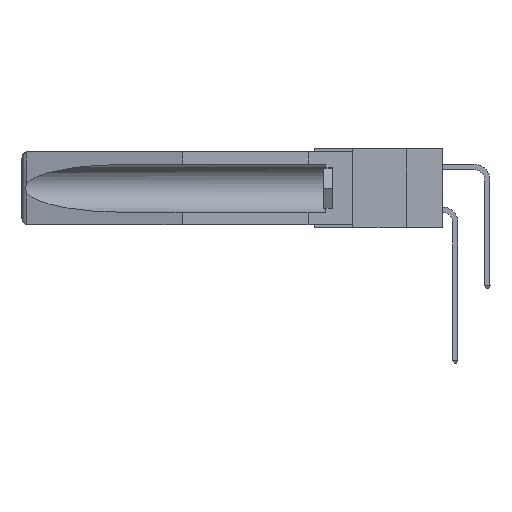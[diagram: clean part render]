
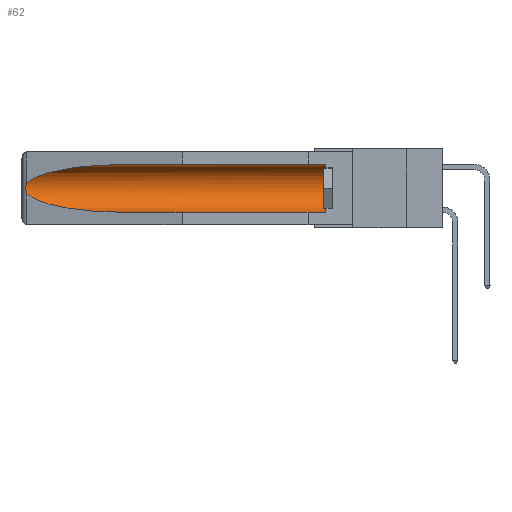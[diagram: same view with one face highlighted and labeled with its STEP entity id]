
A CAD part, left-side view. The second image highlights one B-rep face of the part: STEP entity #62.
In plain terms, the highlighted cylindrical face has radius 2.857 mm (diameter 5.715 mm), a partial arc.
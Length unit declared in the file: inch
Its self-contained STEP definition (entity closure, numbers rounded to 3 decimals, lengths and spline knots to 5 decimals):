
#62 = ADVANCED_FACE ( 'NONE', ( #3431 ), #166, .F. ) ;
#166 = CYLINDRICAL_SURFACE ( 'NONE', #1702, 0.1125 ) ;
#498 = CARTESIAN_POINT ( 'NONE',  ( 0.155, 1.07973, -0.059 ) ) ;
#568 = CARTESIAN_POINT ( 'NONE',  ( 0.25451, 1.48313, -0.09465 ) ) ;
#830 = ORIENTED_EDGE ( 'NONE', *, *, #23297, .T. ) ;
#1090 = ORIENTED_EDGE ( 'NONE', *, *, #8979, .F. ) ;
#1702 = AXIS2_PLACEMENT_3D ( 'NONE', #5433, #23674, #26337 ) ;
#2218 = CIRCLE ( 'NONE', #22630, 0.1125 ) ;
#3092 = VECTOR ( 'NONE', #3189, 39.37008 ) ;
#3189 = DIRECTION ( 'NONE',  ( 0., 1., 0. ) ) ;
#3304 = CARTESIAN_POINT ( 'NONE',  ( 0.26654, 1.53092, -0.15636 ) ) ;
#3431 = FACE_OUTER_BOUND ( 'NONE', #16667, .T. ) ;
#3472 = ORIENTED_EDGE ( 'NONE', *, *, #8042, .T. ) ;
#3806 = CARTESIAN_POINT ( 'NONE',  ( 0.155, 0.126, -0.284 ) ) ;
#5011 = ORIENTED_EDGE ( 'NONE', *, *, #14254, .T. ) ;
#5397 = DIRECTION ( 'NONE',  ( 0., -1., 0. ) ) ;
#5424 = VERTEX_POINT ( 'NONE', #498 ) ;
#5433 = CARTESIAN_POINT ( 'NONE',  ( 0.155, -0.30754, -0.1715 ) ) ;
#6238 = VERTEX_POINT ( 'NONE', #3806 ) ;
#7282 = EDGE_CURVE ( 'NONE', #6238, #15183, #2218, .T. ) ;
#7394 = CARTESIAN_POINT ( 'NONE',  ( 0.2675, 1.53308, -0.17534 ) ) ;
#7435 = CARTESIAN_POINT ( 'NONE',  ( 0.155, 0.126, -0.059 ) ) ;
#7618 = DIRECTION ( 'NONE',  ( 0., 0., 1. ) ) ;
#7759 = CARTESIAN_POINT ( 'NONE',  ( 0.26655, 1.53094, -0.18657 ) ) ;
#8042 = EDGE_CURVE ( 'NONE', #5424, #17426, #20047, .T. ) ;
#8227 = CARTESIAN_POINT ( 'NONE',  ( 0.26537, 1.52718, -0.14972 ) ) ;
#8979 = EDGE_CURVE ( 'NONE', #6238, #10886, #10139, .T. ) ;
#9926 = CARTESIAN_POINT ( 'NONE',  ( 0.26537, 1.52718, -0.19328 ) ) ;
#10139 = LINE ( 'NONE', #11407, #3092 ) ;
#10175 = CARTESIAN_POINT ( 'NONE',  ( 0.155, 1.07973, -0.284 ) ) ;
#10333 = CARTESIAN_POINT ( 'NONE',  ( 0.21114, 1.30732, -0.284 ) ) ;
#10658 = ORIENTED_EDGE ( 'NONE', *, *, #7282, .T. ) ;
#10886 = VERTEX_POINT ( 'NONE', #13370 ) ;
#11407 = CARTESIAN_POINT ( 'NONE',  ( 0.155, -0.30754, -0.284 ) ) ;
#11933 =( BOUNDED_CURVE ( )  B_SPLINE_CURVE ( 3, ( #24404, #22502, #10333, #10175 ),
 .UNSPECIFIED., .F., .F. ) 
 B_SPLINE_CURVE_WITH_KNOTS ( ( 4, 4 ),
 ( 0.1948, 1.5708 ),
 .UNSPECIFIED. ) 
 CURVE ( )  GEOMETRIC_REPRESENTATION_ITEM ( )  RATIONAL_B_SPLINE_CURVE ( ( 1., 0.848, 0.848, 1. ) ) 
 REPRESENTATION_ITEM ( '' )  );
#12112 = VERTEX_POINT ( 'NONE', #9926 ) ;
#12796 = ORIENTED_EDGE ( 'NONE', *, *, #21120, .T. ) ;
#13083 = B_SPLINE_CURVE_WITH_KNOTS ( 'NONE', 3,
 ( #24043, #19747, #3304, #17957, #21881, #7394, #21969, #7759, #25896, #23866 ),
 .UNSPECIFIED., .F., .F.,
 ( 4, 2, 2, 2, 4 ),
 ( 0., 0.00029, 0.00058, 0.00087, 0.00117 ),
 .UNSPECIFIED. ) ;
#13370 = CARTESIAN_POINT ( 'NONE',  ( 0.155, 1.07973, -0.284 ) ) ;
#14254 = EDGE_CURVE ( 'NONE', #12112, #10886, #11933, .T. ) ;
#14937 = CARTESIAN_POINT ( 'NONE',  ( 0.26537, 1.52718, -0.14972 ) ) ;
#15183 = VERTEX_POINT ( 'NONE', #7435 ) ;
#16667 = EDGE_LOOP ( 'NONE', ( #3472, #830, #5011, #1090, #10658, #12796 ) ) ;
#16756 = CARTESIAN_POINT ( 'NONE',  ( 0.155, 1.07973, -0.059 ) ) ;
#16911 = VECTOR ( 'NONE', #26166, 39.37008 ) ;
#17426 = VERTEX_POINT ( 'NONE', #8227 ) ;
#17957 = CARTESIAN_POINT ( 'NONE',  ( 0.2673, 1.5327, -0.16383 ) ) ;
#19747 = CARTESIAN_POINT ( 'NONE',  ( 0.26597, 1.52961, -0.15275 ) ) ;
#20047 =( BOUNDED_CURVE ( )  B_SPLINE_CURVE ( 3, ( #16756, #25010, #568, #14937 ),
 .UNSPECIFIED., .F., .F. ) 
 B_SPLINE_CURVE_WITH_KNOTS ( ( 4, 4 ),
 ( 4.71239, 6.08839 ),
 .UNSPECIFIED. ) 
 CURVE ( )  GEOMETRIC_REPRESENTATION_ITEM ( )  RATIONAL_B_SPLINE_CURVE ( ( 1., 0.848, 0.848, 1. ) ) 
 REPRESENTATION_ITEM ( '' )  );
#21120 = EDGE_CURVE ( 'NONE', #15183, #5424, #23973, .T. ) ;
#21881 = CARTESIAN_POINT ( 'NONE',  ( 0.2675, 1.53308, -0.16763 ) ) ;
#21915 = CARTESIAN_POINT ( 'NONE',  ( 0.155, 0.126, -0.1715 ) ) ;
#21969 = CARTESIAN_POINT ( 'NONE',  ( 0.2673, 1.53269, -0.17917 ) ) ;
#22322 = CARTESIAN_POINT ( 'NONE',  ( 0.155, -0.30754, -0.059 ) ) ;
#22502 = CARTESIAN_POINT ( 'NONE',  ( 0.25451, 1.48313, -0.24835 ) ) ;
#22630 = AXIS2_PLACEMENT_3D ( 'NONE', #21915, #5397, #7618 ) ;
#23297 = EDGE_CURVE ( 'NONE', #17426, #12112, #13083, .T. ) ;
#23674 = DIRECTION ( 'NONE',  ( 0., 1., 0. ) ) ;
#23866 = CARTESIAN_POINT ( 'NONE',  ( 0.26537, 1.52718, -0.19328 ) ) ;
#23973 = LINE ( 'NONE', #22322, #16911 ) ;
#24043 = CARTESIAN_POINT ( 'NONE',  ( 0.26537, 1.52718, -0.14972 ) ) ;
#24404 = CARTESIAN_POINT ( 'NONE',  ( 0.26537, 1.52718, -0.19328 ) ) ;
#25010 = CARTESIAN_POINT ( 'NONE',  ( 0.21114, 1.30732, -0.059 ) ) ;
#25896 = CARTESIAN_POINT ( 'NONE',  ( 0.26597, 1.5296, -0.19026 ) ) ;
#26166 = DIRECTION ( 'NONE',  ( 0., 1., 0. ) ) ;
#26337 = DIRECTION ( 'NONE',  ( 0., 0., 1. ) ) ;
